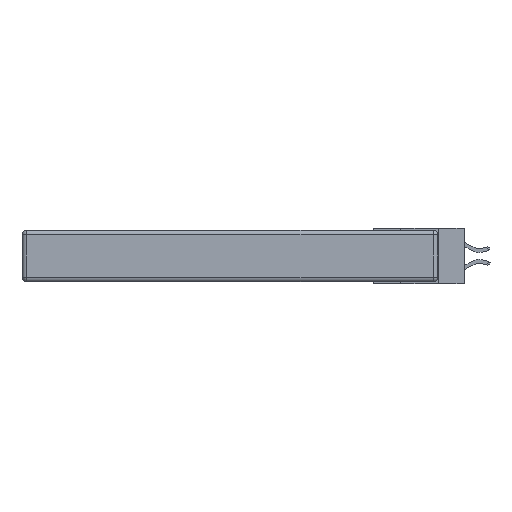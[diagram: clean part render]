
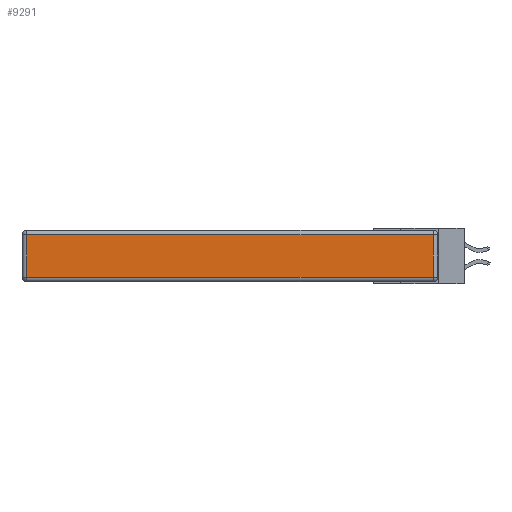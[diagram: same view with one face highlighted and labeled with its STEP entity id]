
A CAD part, left-side view. The second image highlights one B-rep face of the part: STEP entity #9291.
In plain terms, the highlighted planar face has unit normal (-1, 0, 0).
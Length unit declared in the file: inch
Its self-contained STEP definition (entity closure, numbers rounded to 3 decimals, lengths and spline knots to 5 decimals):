
#5192 = EDGE_CURVE ( 'NONE', #31971, #21471, #7613, .T. ) ;
#7613 = LINE ( 'NONE', #29132, #23900 ) ;
#7927 = EDGE_LOOP ( 'NONE', ( #12252, #27136, #32453, #30572 ) ) ;
#8409 = CARTESIAN_POINT ( 'NONE',  ( 0., 0.03, -0.313 ) ) ;
#8547 = PLANE ( 'NONE',  #20489 ) ;
#9291 = ADVANCED_FACE ( 'NONE', ( #25360 ), #8547, .T. ) ;
#9365 = VECTOR ( 'NONE', #31610, 39.37008 ) ;
#10974 = CARTESIAN_POINT ( 'NONE',  ( 0., 2.75, -0.03 ) ) ;
#12252 = ORIENTED_EDGE ( 'NONE', *, *, #22599, .T. ) ;
#14948 = DIRECTION ( 'NONE',  ( 0., 0., -1. ) ) ;
#16008 = LINE ( 'NONE', #28289, #18446 ) ;
#16353 = DIRECTION ( 'NONE',  ( 0., 0., 1. ) ) ;
#17690 = CARTESIAN_POINT ( 'NONE',  ( 0., 0.03, -0.03 ) ) ;
#18446 = VECTOR ( 'NONE', #14948, 39.37008 ) ;
#18798 = DIRECTION ( 'NONE',  ( 0., 0., 1. ) ) ;
#19954 = EDGE_CURVE ( 'NONE', #21471, #20554, #31156, .T. ) ;
#20489 = AXIS2_PLACEMENT_3D ( 'NONE', #24515, #29303, #18798 ) ;
#20521 = VECTOR ( 'NONE', #21303, 39.37008 ) ;
#20554 = VERTEX_POINT ( 'NONE', #20737 ) ;
#20737 = CARTESIAN_POINT ( 'NONE',  ( 0., 2.72, -0.03 ) ) ;
#20815 = EDGE_CURVE ( 'NONE', #20554, #26658, #16008, .T. ) ;
#21303 = DIRECTION ( 'NONE',  ( 0., 1., 0. ) ) ;
#21471 = VERTEX_POINT ( 'NONE', #17690 ) ;
#22599 = EDGE_CURVE ( 'NONE', #26658, #31971, #25717, .T. ) ;
#22817 = CARTESIAN_POINT ( 'NONE',  ( 0., 2.72, -0.313 ) ) ;
#23900 = VECTOR ( 'NONE', #16353, 39.37008 ) ;
#24515 = CARTESIAN_POINT ( 'NONE',  ( 0., 0., -0.343 ) ) ;
#25360 = FACE_OUTER_BOUND ( 'NONE', #7927, .T. ) ;
#25717 = LINE ( 'NONE', #29310, #9365 ) ;
#26658 = VERTEX_POINT ( 'NONE', #22817 ) ;
#27136 = ORIENTED_EDGE ( 'NONE', *, *, #5192, .T. ) ;
#28289 = CARTESIAN_POINT ( 'NONE',  ( 0., 2.72, -0.343 ) ) ;
#29132 = CARTESIAN_POINT ( 'NONE',  ( 0., 0.03, -0.343 ) ) ;
#29303 = DIRECTION ( 'NONE',  ( -1., 0., 0. ) ) ;
#29310 = CARTESIAN_POINT ( 'NONE',  ( 0., 0., -0.313 ) ) ;
#30572 = ORIENTED_EDGE ( 'NONE', *, *, #20815, .T. ) ;
#31156 = LINE ( 'NONE', #10974, #20521 ) ;
#31610 = DIRECTION ( 'NONE',  ( 0., -1., 0. ) ) ;
#31971 = VERTEX_POINT ( 'NONE', #8409 ) ;
#32453 = ORIENTED_EDGE ( 'NONE', *, *, #19954, .T. ) ;
